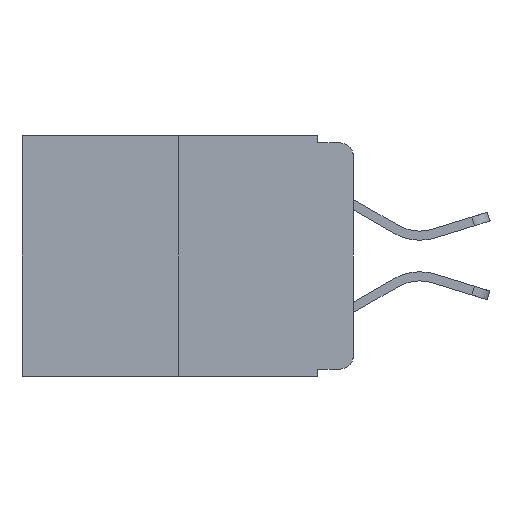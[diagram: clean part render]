
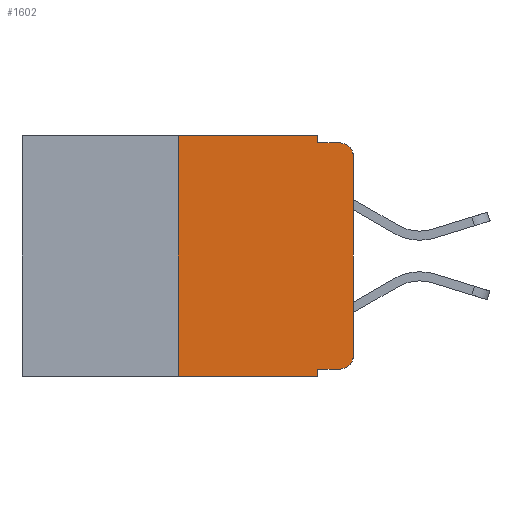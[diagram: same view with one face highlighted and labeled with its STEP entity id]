
A CAD part, left-side view. The second image highlights one B-rep face of the part: STEP entity #1602.
In plain terms, the highlighted planar face has unit normal (-1, 0, 0).
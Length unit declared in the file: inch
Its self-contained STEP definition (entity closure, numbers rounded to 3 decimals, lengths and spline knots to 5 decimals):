
#249 = VECTOR ( 'NONE', #1904, 39.37008 ) ;
#665 = VERTEX_POINT ( 'NONE', #8818 ) ;
#987 = ORIENTED_EDGE ( 'NONE', *, *, #3771, .T. ) ;
#1032 = EDGE_LOOP ( 'NONE', ( #4795, #6218, #7118, #9627, #6470, #5360, #4444, #9873, #11133, #987 ) ) ;
#1132 = LINE ( 'NONE', #2158, #5635 ) ;
#1172 = LINE ( 'NONE', #8615, #10146 ) ;
#1496 = PLANE ( 'NONE',  #4421 ) ;
#1602 = ADVANCED_FACE ( 'NONE', ( #9785 ), #1496, .F. ) ;
#1614 = DIRECTION ( 'NONE',  ( 0., 0., -1. ) ) ;
#1904 = DIRECTION ( 'NONE',  ( 0., -1., 0. ) ) ;
#1965 = CARTESIAN_POINT ( 'NONE',  ( 0., 0., -0.03 ) ) ;
#2155 = VERTEX_POINT ( 'NONE', #7231 ) ;
#2158 = CARTESIAN_POINT ( 'NONE',  ( 0., 0.051, 0. ) ) ;
#2578 = VERTEX_POINT ( 'NONE', #7135 ) ;
#2621 = EDGE_CURVE ( 'NONE', #3707, #9227, #10870, .T. ) ;
#2661 = DIRECTION ( 'NONE',  ( 0., 0., -1. ) ) ;
#2706 = LINE ( 'NONE', #3701, #249 ) ;
#2891 = CARTESIAN_POINT ( 'NONE',  ( 0., 0.051, -0.333 ) ) ;
#3107 = CIRCLE ( 'NONE', #4915, 0.02 ) ;
#3209 = LINE ( 'NONE', #2891, #8095 ) ;
#3345 = DIRECTION ( 'NONE',  ( 0., -1., 0. ) ) ;
#3481 = DIRECTION ( 'NONE',  ( 0., 0., 1. ) ) ;
#3606 = LINE ( 'NONE', #8736, #5654 ) ;
#3701 = CARTESIAN_POINT ( 'NONE',  ( 0., 0.051, -0.01 ) ) ;
#3707 = VERTEX_POINT ( 'NONE', #9546 ) ;
#3771 = EDGE_CURVE ( 'NONE', #9094, #665, #8301, .T. ) ;
#3920 = CARTESIAN_POINT ( 'NONE',  ( 0., 0.02, -0.333 ) ) ;
#4115 = CARTESIAN_POINT ( 'NONE',  ( 0., 0.051, -0.01 ) ) ;
#4174 = VERTEX_POINT ( 'NONE', #1965 ) ;
#4361 = DIRECTION ( 'NONE',  ( 0., 0., -1. ) ) ;
#4421 = AXIS2_PLACEMENT_3D ( 'NONE', #10777, #7895, #10862 ) ;
#4444 = ORIENTED_EDGE ( 'NONE', *, *, #10968, .T. ) ;
#4720 = VECTOR ( 'NONE', #7879, 39.37008 ) ;
#4795 = ORIENTED_EDGE ( 'NONE', *, *, #8827, .T. ) ;
#4915 = AXIS2_PLACEMENT_3D ( 'NONE', #10244, #8668, #1614 ) ;
#4991 = EDGE_CURVE ( 'NONE', #8158, #2155, #1132, .T. ) ;
#5098 = CARTESIAN_POINT ( 'NONE',  ( 0., 0.051, 0. ) ) ;
#5104 = CARTESIAN_POINT ( 'NONE',  ( 0., 0.02, -0.313 ) ) ;
#5184 = CARTESIAN_POINT ( 'NONE',  ( 0., 0.051, -0.333 ) ) ;
#5360 = ORIENTED_EDGE ( 'NONE', *, *, #7842, .F. ) ;
#5596 = EDGE_CURVE ( 'NONE', #9227, #2578, #2706, .T. ) ;
#5635 = VECTOR ( 'NONE', #2661, 39.37008 ) ;
#5654 = VECTOR ( 'NONE', #7932, 39.37008 ) ;
#6109 = CARTESIAN_POINT ( 'NONE',  ( 0., 0.25, 0. ) ) ;
#6180 = EDGE_CURVE ( 'NONE', #4174, #2578, #3107, .T. ) ;
#6218 = ORIENTED_EDGE ( 'NONE', *, *, #6180, .T. ) ;
#6470 = ORIENTED_EDGE ( 'NONE', *, *, #10075, .F. ) ;
#6733 = VECTOR ( 'NONE', #4361, 39.37008 ) ;
#6833 = VECTOR ( 'NONE', #3345, 39.37008 ) ;
#7043 = DIRECTION ( 'NONE',  ( 0., -1., 0. ) ) ;
#7045 = LINE ( 'NONE', #7207, #4720 ) ;
#7118 = ORIENTED_EDGE ( 'NONE', *, *, #5596, .F. ) ;
#7135 = CARTESIAN_POINT ( 'NONE',  ( 0., 0.02, -0.01 ) ) ;
#7207 = CARTESIAN_POINT ( 'NONE',  ( 0., 0.25, 0. ) ) ;
#7231 = CARTESIAN_POINT ( 'NONE',  ( 0., 0.051, -0.343 ) ) ;
#7324 = VERTEX_POINT ( 'NONE', #6109 ) ;
#7325 = CARTESIAN_POINT ( 'NONE',  ( 0., 0.25, -0.343 ) ) ;
#7842 = EDGE_CURVE ( 'NONE', #8041, #7324, #7045, .T. ) ;
#7879 = DIRECTION ( 'NONE',  ( 0., 0., 1. ) ) ;
#7895 = DIRECTION ( 'NONE',  ( 1., 0., 0. ) ) ;
#7932 = DIRECTION ( 'NONE',  ( 0., -1., 0. ) ) ;
#8041 = VERTEX_POINT ( 'NONE', #7325 ) ;
#8095 = VECTOR ( 'NONE', #7043, 39.37008 ) ;
#8158 = VERTEX_POINT ( 'NONE', #5184 ) ;
#8205 = EDGE_CURVE ( 'NONE', #8158, #9094, #3209, .T. ) ;
#8301 = CIRCLE ( 'NONE', #11038, 0.02 ) ;
#8521 = CARTESIAN_POINT ( 'NONE',  ( 0., 0.473, -0.343 ) ) ;
#8615 = CARTESIAN_POINT ( 'NONE',  ( 0., 0., 0. ) ) ;
#8668 = DIRECTION ( 'NONE',  ( -1., 0., 0. ) ) ;
#8736 = CARTESIAN_POINT ( 'NONE',  ( 0., 0.473, 0. ) ) ;
#8818 = CARTESIAN_POINT ( 'NONE',  ( 0., 0., -0.313 ) ) ;
#8827 = EDGE_CURVE ( 'NONE', #665, #4174, #1172, .T. ) ;
#9094 = VERTEX_POINT ( 'NONE', #3920 ) ;
#9227 = VERTEX_POINT ( 'NONE', #4115 ) ;
#9546 = CARTESIAN_POINT ( 'NONE',  ( 0., 0.051, 0. ) ) ;
#9627 = ORIENTED_EDGE ( 'NONE', *, *, #2621, .F. ) ;
#9637 = DIRECTION ( 'NONE',  ( 0., 0., -1. ) ) ;
#9785 = FACE_OUTER_BOUND ( 'NONE', #1032, .T. ) ;
#9873 = ORIENTED_EDGE ( 'NONE', *, *, #4991, .F. ) ;
#10075 = EDGE_CURVE ( 'NONE', #7324, #3707, #3606, .T. ) ;
#10146 = VECTOR ( 'NONE', #3481, 39.37008 ) ;
#10171 = DIRECTION ( 'NONE',  ( -1., 0., 0. ) ) ;
#10244 = CARTESIAN_POINT ( 'NONE',  ( 0., 0.02, -0.03 ) ) ;
#10777 = CARTESIAN_POINT ( 'NONE',  ( 0., 0.473, 0. ) ) ;
#10862 = DIRECTION ( 'NONE',  ( 0., 0., -1. ) ) ;
#10870 = LINE ( 'NONE', #5098, #6733 ) ;
#10968 = EDGE_CURVE ( 'NONE', #8041, #2155, #11203, .T. ) ;
#11038 = AXIS2_PLACEMENT_3D ( 'NONE', #5104, #10171, #9637 ) ;
#11133 = ORIENTED_EDGE ( 'NONE', *, *, #8205, .T. ) ;
#11203 = LINE ( 'NONE', #8521, #6833 ) ;
